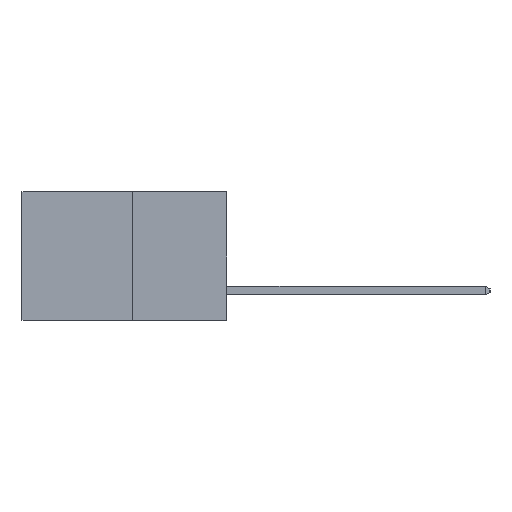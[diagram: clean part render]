
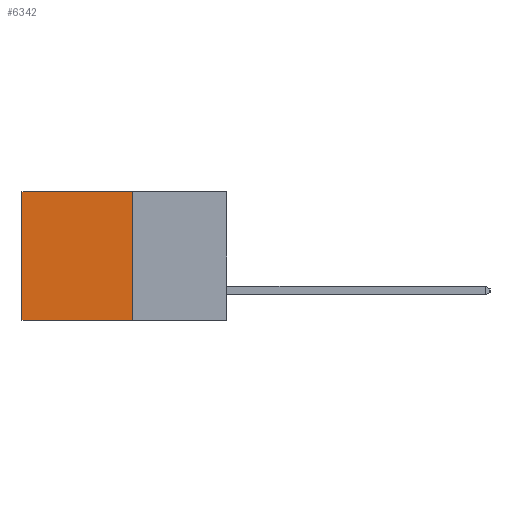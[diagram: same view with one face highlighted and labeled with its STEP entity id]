
A CAD part, left-side view. The second image highlights one B-rep face of the part: STEP entity #6342.
In plain terms, the highlighted planar face has unit normal (-1, 0, 0).
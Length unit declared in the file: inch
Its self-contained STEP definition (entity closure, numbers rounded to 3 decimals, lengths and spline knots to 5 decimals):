
#318 = ORIENTED_EDGE ( 'NONE', *, *, #8710, .F. ) ;
#545 = PLANE ( 'NONE',  #5771 ) ;
#713 = FACE_OUTER_BOUND ( 'NONE', #5571, .T. ) ;
#1140 = LINE ( 'NONE', #4596, #9391 ) ;
#1378 = DIRECTION ( 'NONE',  ( 0., 0., -1. ) ) ;
#1380 = VECTOR ( 'NONE', #5449, 39.37008 ) ;
#1522 = VERTEX_POINT ( 'NONE', #8631 ) ;
#1527 = VECTOR ( 'NONE', #6235, 39.37008 ) ;
#2466 = VERTEX_POINT ( 'NONE', #7861 ) ;
#3600 = LINE ( 'NONE', #6227, #1380 ) ;
#4319 = CARTESIAN_POINT ( 'NONE',  ( 0.277, 0.59, 0. ) ) ;
#4452 = EDGE_CURVE ( 'NONE', #5108, #9359, #1140, .T. ) ;
#4544 = ORIENTED_EDGE ( 'NONE', *, *, #5075, .T. ) ;
#4596 = CARTESIAN_POINT ( 'NONE',  ( 0.277, 0.27, 0. ) ) ;
#4700 = LINE ( 'NONE', #8350, #10400 ) ;
#4707 = CARTESIAN_POINT ( 'NONE',  ( 0.277, 0.27, -0.37 ) ) ;
#5075 = EDGE_CURVE ( 'NONE', #9359, #2466, #9993, .T. ) ;
#5108 = VERTEX_POINT ( 'NONE', #7105 ) ;
#5449 = DIRECTION ( 'NONE',  ( 0., 0., -1. ) ) ;
#5571 = EDGE_LOOP ( 'NONE', ( #4544, #318, #7852, #10482 ) ) ;
#5604 = EDGE_CURVE ( 'NONE', #5108, #1522, #3600, .T. ) ;
#5771 = AXIS2_PLACEMENT_3D ( 'NONE', #4707, #6358, #1378 ) ;
#5892 = DIRECTION ( 'NONE',  ( 0., 1., 0. ) ) ;
#6227 = CARTESIAN_POINT ( 'NONE',  ( 0.277, 0.27, -0.37 ) ) ;
#6235 = DIRECTION ( 'NONE',  ( 0., 0., -1. ) ) ;
#6250 = DIRECTION ( 'NONE',  ( 0., 1., 0. ) ) ;
#6342 = ADVANCED_FACE ( 'NONE', ( #713 ), #545, .F. ) ;
#6358 = DIRECTION ( 'NONE',  ( 1., 0., 0. ) ) ;
#7105 = CARTESIAN_POINT ( 'NONE',  ( 0.277, 0.27, 0. ) ) ;
#7852 = ORIENTED_EDGE ( 'NONE', *, *, #5604, .F. ) ;
#7861 = CARTESIAN_POINT ( 'NONE',  ( 0.277, 0.59, -0.37 ) ) ;
#8350 = CARTESIAN_POINT ( 'NONE',  ( 0.277, 0.27, -0.37 ) ) ;
#8631 = CARTESIAN_POINT ( 'NONE',  ( 0.277, 0.27, -0.37 ) ) ;
#8710 = EDGE_CURVE ( 'NONE', #1522, #2466, #4700, .T. ) ;
#9359 = VERTEX_POINT ( 'NONE', #4319 ) ;
#9391 = VECTOR ( 'NONE', #6250, 39.37008 ) ;
#9993 = LINE ( 'NONE', #10251, #1527 ) ;
#10251 = CARTESIAN_POINT ( 'NONE',  ( 0.277, 0.59, -0.37 ) ) ;
#10400 = VECTOR ( 'NONE', #5892, 39.37008 ) ;
#10482 = ORIENTED_EDGE ( 'NONE', *, *, #4452, .T. ) ;
